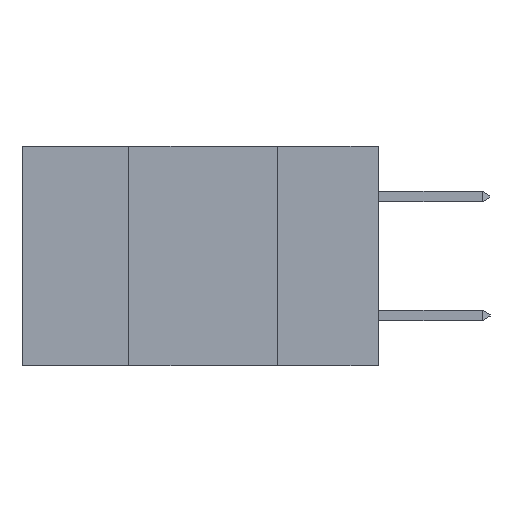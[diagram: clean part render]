
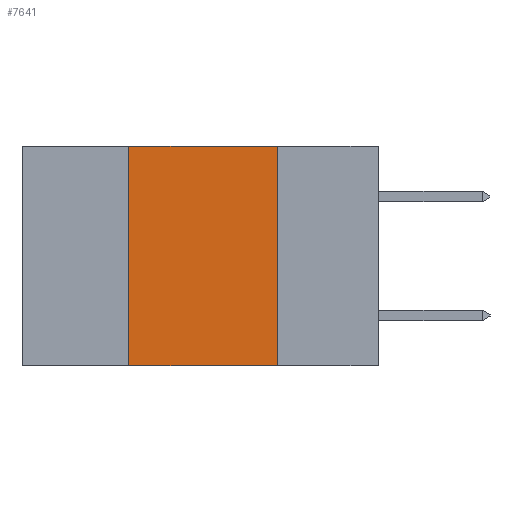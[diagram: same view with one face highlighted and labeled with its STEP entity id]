
A CAD part, left-side view. The second image highlights one B-rep face of the part: STEP entity #7641.
In plain terms, the highlighted planar face has unit normal (-1, 0, 0).
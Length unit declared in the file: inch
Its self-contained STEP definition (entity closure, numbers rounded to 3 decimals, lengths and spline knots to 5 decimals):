
#126 = DIRECTION ( 'NONE',  ( 1., 0., 0. ) ) ;
#351 = VECTOR ( 'NONE', #10903, 39.37008 ) ;
#757 = CARTESIAN_POINT ( 'NONE',  ( 0., 0.6, 0. ) ) ;
#2487 = VERTEX_POINT ( 'NONE', #6859 ) ;
#2570 = CARTESIAN_POINT ( 'NONE',  ( 0., 0.17, -0.37 ) ) ;
#2866 = DIRECTION ( 'NONE',  ( 0., 0., -1. ) ) ;
#3082 = CARTESIAN_POINT ( 'NONE',  ( 0., 0.6, 0. ) ) ;
#3480 = ORIENTED_EDGE ( 'NONE', *, *, #15689, .F. ) ;
#3515 = VECTOR ( 'NONE', #4372, 39.37008 ) ;
#3960 = ORIENTED_EDGE ( 'NONE', *, *, #11916, .T. ) ;
#4316 = CARTESIAN_POINT ( 'NONE',  ( 0., 0.17, -0.37 ) ) ;
#4372 = DIRECTION ( 'NONE',  ( 0., 0., 1. ) ) ;
#6045 = VERTEX_POINT ( 'NONE', #17356 ) ;
#6473 = LINE ( 'NONE', #15698, #3515 ) ;
#6679 = FACE_OUTER_BOUND ( 'NONE', #11790, .T. ) ;
#6859 = CARTESIAN_POINT ( 'NONE',  ( 0., 0.42, 0. ) ) ;
#7351 = PLANE ( 'NONE',  #14786 ) ;
#7641 = ADVANCED_FACE ( 'NONE', ( #6679 ), #7351, .F. ) ;
#7763 = VERTEX_POINT ( 'NONE', #2570 ) ;
#8010 = DIRECTION ( 'NONE',  ( 0., -1., 0. ) ) ;
#10903 = DIRECTION ( 'NONE',  ( 0., -1., 0. ) ) ;
#11148 = DIRECTION ( 'NONE',  ( 0., 0., -1. ) ) ;
#11790 = EDGE_LOOP ( 'NONE', ( #3480, #14847, #18521, #3960 ) ) ;
#11855 = CARTESIAN_POINT ( 'NONE',  ( 0., 0.42, -0.37 ) ) ;
#11916 = EDGE_CURVE ( 'NONE', #17119, #7763, #14057, .T. ) ;
#12858 = EDGE_CURVE ( 'NONE', #17119, #2487, #6473, .T. ) ;
#14057 = LINE ( 'NONE', #16443, #17322 ) ;
#14332 = VECTOR ( 'NONE', #2866, 39.37008 ) ;
#14755 = EDGE_CURVE ( 'NONE', #2487, #6045, #15696, .T. ) ;
#14783 = LINE ( 'NONE', #4316, #14332 ) ;
#14786 = AXIS2_PLACEMENT_3D ( 'NONE', #3082, #126, #11148 ) ;
#14847 = ORIENTED_EDGE ( 'NONE', *, *, #14755, .F. ) ;
#15689 = EDGE_CURVE ( 'NONE', #6045, #7763, #14783, .T. ) ;
#15696 = LINE ( 'NONE', #757, #351 ) ;
#15698 = CARTESIAN_POINT ( 'NONE',  ( 0., 0.42, -0.37 ) ) ;
#16443 = CARTESIAN_POINT ( 'NONE',  ( 0., 0.6, -0.37 ) ) ;
#17119 = VERTEX_POINT ( 'NONE', #11855 ) ;
#17322 = VECTOR ( 'NONE', #8010, 39.37008 ) ;
#17356 = CARTESIAN_POINT ( 'NONE',  ( 0., 0.17, 0. ) ) ;
#18521 = ORIENTED_EDGE ( 'NONE', *, *, #12858, .F. ) ;
